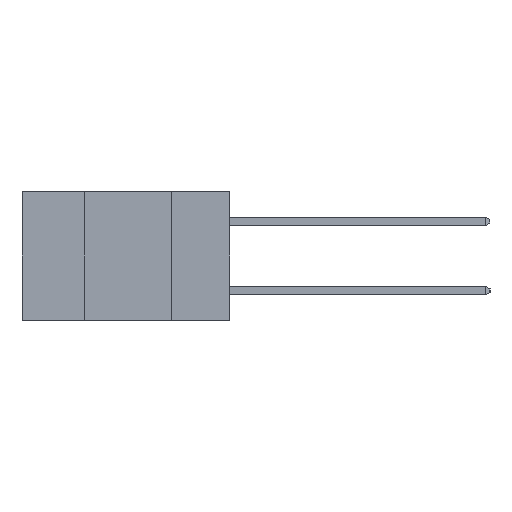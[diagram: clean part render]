
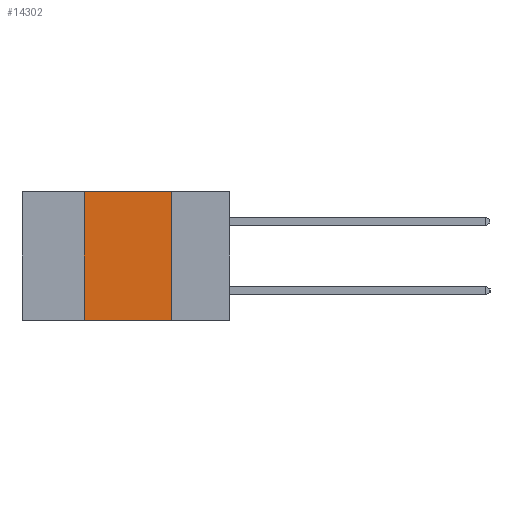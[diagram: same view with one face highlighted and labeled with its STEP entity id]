
A CAD part, left-side view. The second image highlights one B-rep face of the part: STEP entity #14302.
In plain terms, the highlighted planar face has unit normal (-1, 0, 0).
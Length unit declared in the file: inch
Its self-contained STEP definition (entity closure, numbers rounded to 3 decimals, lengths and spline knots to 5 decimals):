
#832 = EDGE_CURVE ( 'NONE', #6692, #14833, #14052, .T. ) ;
#1222 = DIRECTION ( 'NONE',  ( 0., -1., 0. ) ) ;
#1630 = EDGE_CURVE ( 'NONE', #14833, #8931, #14895, .T. ) ;
#2009 = CARTESIAN_POINT ( 'NONE',  ( 0., 0.6, 0. ) ) ;
#2464 = EDGE_CURVE ( 'NONE', #8931, #7933, #3981, .T. ) ;
#2863 = ORIENTED_EDGE ( 'NONE', *, *, #832, .F. ) ;
#3398 = LINE ( 'NONE', #14497, #12783 ) ;
#3981 = LINE ( 'NONE', #9458, #4757 ) ;
#4714 = CARTESIAN_POINT ( 'NONE',  ( 0., 0.42, 0. ) ) ;
#4718 = CARTESIAN_POINT ( 'NONE',  ( 0., 0.17, -0.37 ) ) ;
#4757 = VECTOR ( 'NONE', #9406, 39.37008 ) ;
#5547 = VECTOR ( 'NONE', #9483, 39.37008 ) ;
#6516 = EDGE_LOOP ( 'NONE', ( #14097, #11626, #2863, #10363 ) ) ;
#6692 = VERTEX_POINT ( 'NONE', #14076 ) ;
#7517 = DIRECTION ( 'NONE',  ( 0., 0., -1. ) ) ;
#7933 = VERTEX_POINT ( 'NONE', #4718 ) ;
#8694 = DIRECTION ( 'NONE',  ( 1., 0., 0. ) ) ;
#8931 = VERTEX_POINT ( 'NONE', #13601 ) ;
#9406 = DIRECTION ( 'NONE',  ( 0., 0., -1. ) ) ;
#9458 = CARTESIAN_POINT ( 'NONE',  ( 0., 0.17, -0.37 ) ) ;
#9483 = DIRECTION ( 'NONE',  ( 0., 0., 1. ) ) ;
#9659 = CARTESIAN_POINT ( 'NONE',  ( 0., 0.42, -0.37 ) ) ;
#10363 = ORIENTED_EDGE ( 'NONE', *, *, #14163, .T. ) ;
#10506 = FACE_OUTER_BOUND ( 'NONE', #6516, .T. ) ;
#11589 = CARTESIAN_POINT ( 'NONE',  ( 0., 0.6, 0. ) ) ;
#11626 = ORIENTED_EDGE ( 'NONE', *, *, #1630, .F. ) ;
#12783 = VECTOR ( 'NONE', #14481, 39.37008 ) ;
#13342 = VECTOR ( 'NONE', #1222, 39.37008 ) ;
#13601 = CARTESIAN_POINT ( 'NONE',  ( 0., 0.17, 0. ) ) ;
#13663 = AXIS2_PLACEMENT_3D ( 'NONE', #11589, #8694, #7517 ) ;
#14052 = LINE ( 'NONE', #9659, #5547 ) ;
#14076 = CARTESIAN_POINT ( 'NONE',  ( 0., 0.42, -0.37 ) ) ;
#14097 = ORIENTED_EDGE ( 'NONE', *, *, #2464, .F. ) ;
#14163 = EDGE_CURVE ( 'NONE', #6692, #7933, #3398, .T. ) ;
#14302 = ADVANCED_FACE ( 'NONE', ( #10506 ), #15371, .F. ) ;
#14481 = DIRECTION ( 'NONE',  ( 0., -1., 0. ) ) ;
#14497 = CARTESIAN_POINT ( 'NONE',  ( 0., 0.6, -0.37 ) ) ;
#14833 = VERTEX_POINT ( 'NONE', #4714 ) ;
#14895 = LINE ( 'NONE', #2009, #13342 ) ;
#15371 = PLANE ( 'NONE',  #13663 ) ;
